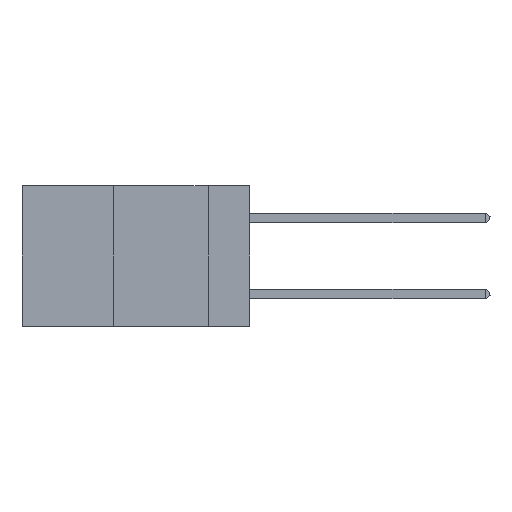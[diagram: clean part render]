
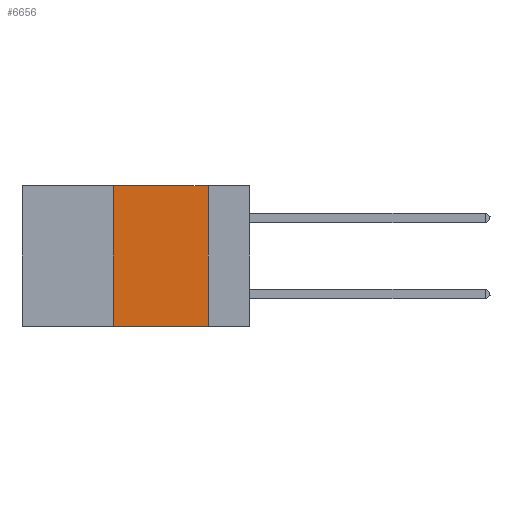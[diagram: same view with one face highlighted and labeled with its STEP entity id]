
A CAD part, left-side view. The second image highlights one B-rep face of the part: STEP entity #6656.
In plain terms, the highlighted planar face has unit normal (-1, 0, 0).
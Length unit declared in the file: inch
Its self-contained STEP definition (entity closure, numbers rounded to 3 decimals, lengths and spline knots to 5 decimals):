
#173 = VECTOR ( 'NONE', #29731, 39.37008 ) ;
#1597 = CARTESIAN_POINT ( 'NONE',  ( 0., 0.36, -0.37 ) ) ;
#1978 = EDGE_CURVE ( 'NONE', #4162, #17633, #12882, .T. ) ;
#2703 = CARTESIAN_POINT ( 'NONE',  ( 0., 0.6, 0. ) ) ;
#3533 = DIRECTION ( 'NONE',  ( 1., 0., 0. ) ) ;
#3704 = AXIS2_PLACEMENT_3D ( 'NONE', #34334, #3533, #25148 ) ;
#3741 = VERTEX_POINT ( 'NONE', #33793 ) ;
#4162 = VERTEX_POINT ( 'NONE', #1597 ) ;
#4926 = LINE ( 'NONE', #10546, #36881 ) ;
#5829 = DIRECTION ( 'NONE',  ( 0., -1., 0. ) ) ;
#5861 = CARTESIAN_POINT ( 'NONE',  ( 0., 0.11, -0.37 ) ) ;
#6609 = VECTOR ( 'NONE', #9397, 39.37008 ) ;
#6656 = ADVANCED_FACE ( 'NONE', ( #33782 ), #12754, .F. ) ;
#6734 = ORIENTED_EDGE ( 'NONE', *, *, #7296, .F. ) ;
#7296 = EDGE_CURVE ( 'NONE', #17633, #3741, #24063, .T. ) ;
#9397 = DIRECTION ( 'NONE',  ( 0., 0., 1. ) ) ;
#10546 = CARTESIAN_POINT ( 'NONE',  ( 0., 0.11, 0. ) ) ;
#10936 = ORIENTED_EDGE ( 'NONE', *, *, #24985, .T. ) ;
#12754 = PLANE ( 'NONE',  #3704 ) ;
#12882 = LINE ( 'NONE', #21282, #6609 ) ;
#14348 = ORIENTED_EDGE ( 'NONE', *, *, #1978, .F. ) ;
#16195 = CARTESIAN_POINT ( 'NONE',  ( 0., 0.36, 0. ) ) ;
#16742 = DIRECTION ( 'NONE',  ( 0., 0., -1. ) ) ;
#17633 = VERTEX_POINT ( 'NONE', #16195 ) ;
#20979 = CARTESIAN_POINT ( 'NONE',  ( 0., 0.6, -0.37 ) ) ;
#21200 = ORIENTED_EDGE ( 'NONE', *, *, #33900, .F. ) ;
#21282 = CARTESIAN_POINT ( 'NONE',  ( 0., 0.36, 0. ) ) ;
#23429 = LINE ( 'NONE', #20979, #173 ) ;
#24063 = LINE ( 'NONE', #2703, #33714 ) ;
#24985 = EDGE_CURVE ( 'NONE', #4162, #32145, #23429, .T. ) ;
#25148 = DIRECTION ( 'NONE',  ( 0., 0., -1. ) ) ;
#29731 = DIRECTION ( 'NONE',  ( 0., -1., 0. ) ) ;
#32145 = VERTEX_POINT ( 'NONE', #5861 ) ;
#32833 = EDGE_LOOP ( 'NONE', ( #21200, #6734, #14348, #10936 ) ) ;
#33714 = VECTOR ( 'NONE', #5829, 39.37008 ) ;
#33782 = FACE_OUTER_BOUND ( 'NONE', #32833, .T. ) ;
#33793 = CARTESIAN_POINT ( 'NONE',  ( 0., 0.11, 0. ) ) ;
#33900 = EDGE_CURVE ( 'NONE', #3741, #32145, #4926, .T. ) ;
#34334 = CARTESIAN_POINT ( 'NONE',  ( 0., 0.6, 0. ) ) ;
#36881 = VECTOR ( 'NONE', #16742, 39.37008 ) ;
